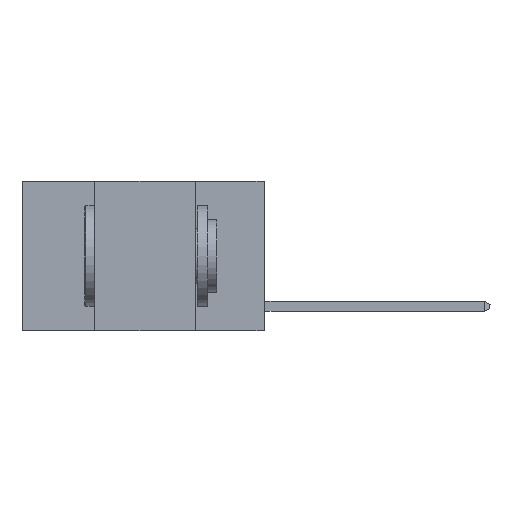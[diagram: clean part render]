
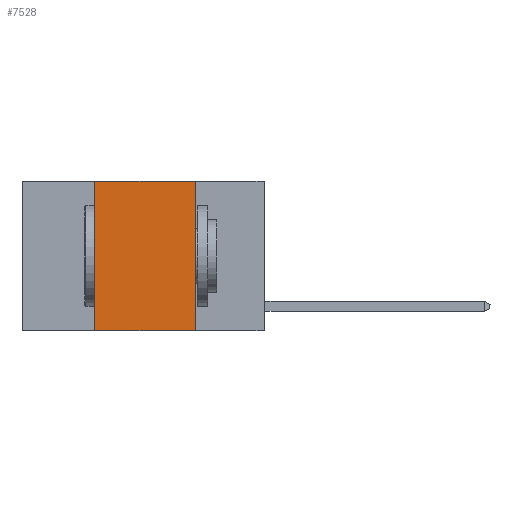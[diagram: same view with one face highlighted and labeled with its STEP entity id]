
A CAD part, left-side view. The second image highlights one B-rep face of the part: STEP entity #7528.
In plain terms, the highlighted planar face has unit normal (-1, 0, 0).
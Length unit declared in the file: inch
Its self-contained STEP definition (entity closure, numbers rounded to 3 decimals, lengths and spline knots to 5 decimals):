
#4 = VECTOR ( 'NONE', #21641, 39.37008 ) ;
#1468 = VECTOR ( 'NONE', #19322, 39.37008 ) ;
#1673 = CARTESIAN_POINT ( 'NONE',  ( 0., 0.42, 0. ) ) ;
#3314 = CARTESIAN_POINT ( 'NONE',  ( 0., 0.6, -0.37 ) ) ;
#3702 = VECTOR ( 'NONE', #9431, 39.37008 ) ;
#3750 = EDGE_CURVE ( 'NONE', #11507, #13935, #8674, .T. ) ;
#4367 = PLANE ( 'NONE',  #19214 ) ;
#5540 = VERTEX_POINT ( 'NONE', #23481 ) ;
#6260 = DIRECTION ( 'NONE',  ( 0., 0., -1. ) ) ;
#7528 = ADVANCED_FACE ( 'NONE', ( #22477 ), #4367, .F. ) ;
#8674 = LINE ( 'NONE', #13133, #3702 ) ;
#9431 = DIRECTION ( 'NONE',  ( 0., 0., -1. ) ) ;
#9994 = ORIENTED_EDGE ( 'NONE', *, *, #3750, .F. ) ;
#10028 = LINE ( 'NONE', #14305, #4 ) ;
#10321 = ORIENTED_EDGE ( 'NONE', *, *, #22544, .F. ) ;
#10935 = EDGE_CURVE ( 'NONE', #5540, #15026, #17570, .T. ) ;
#11507 = VERTEX_POINT ( 'NONE', #18975 ) ;
#11597 = ORIENTED_EDGE ( 'NONE', *, *, #10935, .F. ) ;
#11663 = ORIENTED_EDGE ( 'NONE', *, *, #21282, .T. ) ;
#13133 = CARTESIAN_POINT ( 'NONE',  ( 0., 0.17, 0. ) ) ;
#13484 = CARTESIAN_POINT ( 'NONE',  ( 0., 0.17, -0.37 ) ) ;
#13791 = CARTESIAN_POINT ( 'NONE',  ( 0., 0.42, 0. ) ) ;
#13935 = VERTEX_POINT ( 'NONE', #13484 ) ;
#14305 = CARTESIAN_POINT ( 'NONE',  ( 0., 0.6, 0. ) ) ;
#15026 = VERTEX_POINT ( 'NONE', #1673 ) ;
#15046 = LINE ( 'NONE', #3314, #15641 ) ;
#15593 = CARTESIAN_POINT ( 'NONE',  ( 0., 0.6, 0. ) ) ;
#15641 = VECTOR ( 'NONE', #16412, 39.37008 ) ;
#16412 = DIRECTION ( 'NONE',  ( 0., -1., 0. ) ) ;
#17446 = DIRECTION ( 'NONE',  ( 1., 0., 0. ) ) ;
#17570 = LINE ( 'NONE', #13791, #1468 ) ;
#18975 = CARTESIAN_POINT ( 'NONE',  ( 0., 0.17, 0. ) ) ;
#19214 = AXIS2_PLACEMENT_3D ( 'NONE', #15593, #17446, #6260 ) ;
#19322 = DIRECTION ( 'NONE',  ( 0., 0., 1. ) ) ;
#21282 = EDGE_CURVE ( 'NONE', #5540, #13935, #15046, .T. ) ;
#21641 = DIRECTION ( 'NONE',  ( 0., -1., 0. ) ) ;
#22477 = FACE_OUTER_BOUND ( 'NONE', #23056, .T. ) ;
#22544 = EDGE_CURVE ( 'NONE', #15026, #11507, #10028, .T. ) ;
#23056 = EDGE_LOOP ( 'NONE', ( #9994, #10321, #11597, #11663 ) ) ;
#23481 = CARTESIAN_POINT ( 'NONE',  ( 0., 0.42, -0.37 ) ) ;
